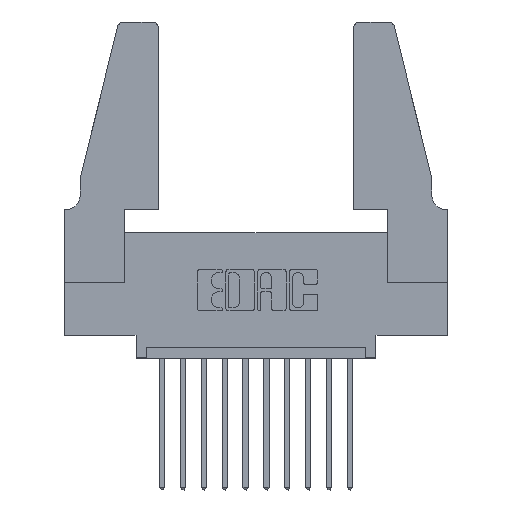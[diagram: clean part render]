
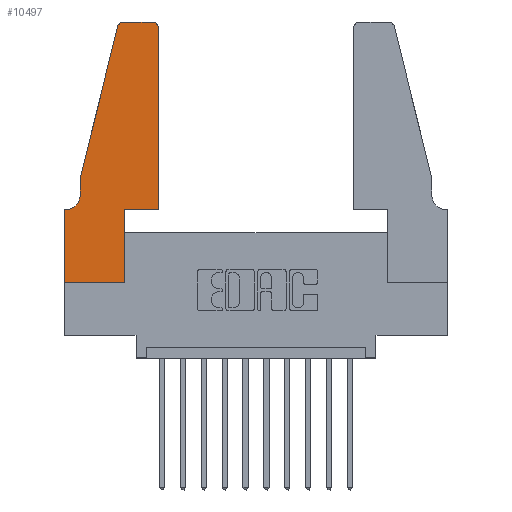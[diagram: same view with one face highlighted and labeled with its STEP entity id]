
A CAD part, top view. The second image highlights one B-rep face of the part: STEP entity #10497.
In plain terms, the highlighted planar face has unit normal (0, 0, 1).
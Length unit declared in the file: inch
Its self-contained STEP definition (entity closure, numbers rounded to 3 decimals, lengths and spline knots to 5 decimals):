
#153 = PLANE ( 'NONE',  #3836 ) ;
#181 = VERTEX_POINT ( 'NONE', #9110 ) ;
#348 = VERTEX_POINT ( 'NONE', #4529 ) ;
#361 = DIRECTION ( 'NONE',  ( 1., 0., 0. ) ) ;
#649 = DIRECTION ( 'NONE',  ( 0., -1., 0. ) ) ;
#734 = LINE ( 'NONE', #3218, #8589 ) ;
#907 = CARTESIAN_POINT ( 'NONE',  ( 0., 0., 0.37 ) ) ;
#1113 = EDGE_LOOP ( 'NONE', ( #7995, #12048, #8029, #8327, #5014, #5134, #14109, #6977, #10657, #8624, #7728, #1678 ) ) ;
#1229 = VECTOR ( 'NONE', #7771, 39.37008 ) ;
#1270 = CARTESIAN_POINT ( 'NONE',  ( 0., 0.35, 0.37 ) ) ;
#1297 = EDGE_CURVE ( 'NONE', #348, #7904, #1729, .T. ) ;
#1383 = VERTEX_POINT ( 'NONE', #4449 ) ;
#1439 = EDGE_CURVE ( 'NONE', #13309, #4636, #9750, .T. ) ;
#1475 = CARTESIAN_POINT ( 'NONE',  ( 0.4205, 1.25, 0.37 ) ) ;
#1489 = AXIS2_PLACEMENT_3D ( 'NONE', #8717, #2160, #9809 ) ;
#1678 = ORIENTED_EDGE ( 'NONE', *, *, #8527, .T. ) ;
#1729 = CIRCLE ( 'NONE', #1489, 0.07 ) ;
#1959 = CARTESIAN_POINT ( 'NONE',  ( 0.2605, 1.25, 0.37 ) ) ;
#2160 = DIRECTION ( 'NONE',  ( 0., 0., -1. ) ) ;
#2265 = AXIS2_PLACEMENT_3D ( 'NONE', #3436, #7798, #361 ) ;
#2539 = VECTOR ( 'NONE', #4648, 39.37008 ) ;
#3090 = VECTOR ( 'NONE', #8146, 39.37008 ) ;
#3218 = CARTESIAN_POINT ( 'NONE',  ( 0.2865, 0.35, 0.37 ) ) ;
#3329 = VERTEX_POINT ( 'NONE', #6638 ) ;
#3348 = CARTESIAN_POINT ( 'NONE',  ( 0., 0., 0.37 ) ) ;
#3436 = CARTESIAN_POINT ( 'NONE',  ( 0.4205, 1.22, 0.37 ) ) ;
#3503 = VECTOR ( 'NONE', #11050, 39.37008 ) ;
#3537 = CARTESIAN_POINT ( 'NONE',  ( 0.0755, 0.35, 0.37 ) ) ;
#3575 = LINE ( 'NONE', #3537, #2539 ) ;
#3617 = VERTEX_POINT ( 'NONE', #13131 ) ;
#3804 = VECTOR ( 'NONE', #9212, 39.37008 ) ;
#3836 = AXIS2_PLACEMENT_3D ( 'NONE', #1270, #4457, #8918 ) ;
#3867 = VERTEX_POINT ( 'NONE', #5359 ) ;
#4449 = CARTESIAN_POINT ( 'NONE',  ( 0.4505, 0.35, 0.37 ) ) ;
#4457 = DIRECTION ( 'NONE',  ( 0., 0., 1. ) ) ;
#4529 = CARTESIAN_POINT ( 'NONE',  ( 0.0755, 0.42, 0.37 ) ) ;
#4636 = VERTEX_POINT ( 'NONE', #9438 ) ;
#4648 = DIRECTION ( 'NONE',  ( -1., 0., 0. ) ) ;
#4811 = LINE ( 'NONE', #11480, #12326 ) ;
#5014 = ORIENTED_EDGE ( 'NONE', *, *, #1297, .T. ) ;
#5134 = ORIENTED_EDGE ( 'NONE', *, *, #10176, .T. ) ;
#5359 = CARTESIAN_POINT ( 'NONE',  ( 0.2865, 0.35, 0.37 ) ) ;
#5570 = CARTESIAN_POINT ( 'NONE',  ( 0.0755, 0.5, 0.37 ) ) ;
#5746 = EDGE_CURVE ( 'NONE', #9471, #3617, #8341, .T. ) ;
#5829 = EDGE_CURVE ( 'NONE', #9711, #9471, #8157, .T. ) ;
#5863 = EDGE_CURVE ( 'NONE', #11238, #13309, #10684, .T. ) ;
#6517 = DIRECTION ( 'NONE',  ( 0., -1., 0. ) ) ;
#6638 = CARTESIAN_POINT ( 'NONE',  ( 0.4505, 1.22, 0.37 ) ) ;
#6731 = LINE ( 'NONE', #9120, #3804 ) ;
#6977 = ORIENTED_EDGE ( 'NONE', *, *, #1439, .T. ) ;
#7017 = EDGE_CURVE ( 'NONE', #3617, #181, #8315, .T. ) ;
#7287 = DIRECTION ( 'NONE',  ( 1., 0., 0. ) ) ;
#7401 = CARTESIAN_POINT ( 'NONE',  ( 0., 0.35, 0.37 ) ) ;
#7728 = ORIENTED_EDGE ( 'NONE', *, *, #11634, .T. ) ;
#7771 = DIRECTION ( 'NONE',  ( 1., 0., 0. ) ) ;
#7798 = DIRECTION ( 'NONE',  ( 0., 0., 1. ) ) ;
#7818 = VECTOR ( 'NONE', #6517, 39.37008 ) ;
#7904 = VERTEX_POINT ( 'NONE', #11426 ) ;
#7995 = ORIENTED_EDGE ( 'NONE', *, *, #5829, .T. ) ;
#8029 = ORIENTED_EDGE ( 'NONE', *, *, #7017, .T. ) ;
#8146 = DIRECTION ( 'NONE',  ( 1., 0., 0. ) ) ;
#8157 = LINE ( 'NONE', #1959, #9852 ) ;
#8315 = LINE ( 'NONE', #5570, #3503 ) ;
#8327 = ORIENTED_EDGE ( 'NONE', *, *, #9731, .T. ) ;
#8341 = CIRCLE ( 'NONE', #9479, 0.03 ) ;
#8427 = CIRCLE ( 'NONE', #2265, 0.03 ) ;
#8449 = EDGE_CURVE ( 'NONE', #4636, #3867, #734, .T. ) ;
#8527 = EDGE_CURVE ( 'NONE', #3329, #9711, #8427, .T. ) ;
#8589 = VECTOR ( 'NONE', #8968, 39.37008 ) ;
#8612 = EDGE_CURVE ( 'NONE', #3867, #1383, #12013, .T. ) ;
#8624 = ORIENTED_EDGE ( 'NONE', *, *, #8612, .T. ) ;
#8717 = CARTESIAN_POINT ( 'NONE',  ( 0.0055, 0.42, 0.37 ) ) ;
#8918 = DIRECTION ( 'NONE',  ( 1., 0., 0. ) ) ;
#8968 = DIRECTION ( 'NONE',  ( 0., 1., 0. ) ) ;
#9110 = CARTESIAN_POINT ( 'NONE',  ( 0.0755, 0.5, 0.37 ) ) ;
#9120 = CARTESIAN_POINT ( 'NONE',  ( 0.4505, 0.35, 0.37 ) ) ;
#9212 = DIRECTION ( 'NONE',  ( 0., 1., 0. ) ) ;
#9438 = CARTESIAN_POINT ( 'NONE',  ( 0.2865, 0., 0.37 ) ) ;
#9471 = VERTEX_POINT ( 'NONE', #11413 ) ;
#9479 = AXIS2_PLACEMENT_3D ( 'NONE', #13777, #10417, #7287 ) ;
#9605 = DIRECTION ( 'NONE',  ( -1., 0., 0. ) ) ;
#9711 = VERTEX_POINT ( 'NONE', #1475 ) ;
#9731 = EDGE_CURVE ( 'NONE', #181, #348, #4811, .T. ) ;
#9750 = LINE ( 'NONE', #3348, #1229 ) ;
#9809 = DIRECTION ( 'NONE',  ( -1., 0., 0. ) ) ;
#9852 = VECTOR ( 'NONE', #9605, 39.37008 ) ;
#10176 = EDGE_CURVE ( 'NONE', #7904, #11238, #3575, .T. ) ;
#10417 = DIRECTION ( 'NONE',  ( 0., 0., 1. ) ) ;
#10497 = ADVANCED_FACE ( 'NONE', ( #11945 ), #153, .T. ) ;
#10657 = ORIENTED_EDGE ( 'NONE', *, *, #8449, .T. ) ;
#10684 = LINE ( 'NONE', #10824, #7818 ) ;
#10824 = CARTESIAN_POINT ( 'NONE',  ( 0., 0., 0.37 ) ) ;
#11050 = DIRECTION ( 'NONE',  ( -0.239, -0.971, 0. ) ) ;
#11238 = VERTEX_POINT ( 'NONE', #7401 ) ;
#11413 = CARTESIAN_POINT ( 'NONE',  ( 0.284, 1.25, 0.37 ) ) ;
#11426 = CARTESIAN_POINT ( 'NONE',  ( 0.0055, 0.35, 0.37 ) ) ;
#11437 = CARTESIAN_POINT ( 'NONE',  ( 0.4505, 0.35, 0.37 ) ) ;
#11480 = CARTESIAN_POINT ( 'NONE',  ( 0.0755, 0.5, 0.37 ) ) ;
#11634 = EDGE_CURVE ( 'NONE', #1383, #3329, #6731, .T. ) ;
#11945 = FACE_OUTER_BOUND ( 'NONE', #1113, .T. ) ;
#12013 = LINE ( 'NONE', #11437, #3090 ) ;
#12048 = ORIENTED_EDGE ( 'NONE', *, *, #5746, .T. ) ;
#12326 = VECTOR ( 'NONE', #649, 39.37008 ) ;
#13131 = CARTESIAN_POINT ( 'NONE',  ( 0.25487, 1.22718, 0.37 ) ) ;
#13309 = VERTEX_POINT ( 'NONE', #907 ) ;
#13777 = CARTESIAN_POINT ( 'NONE',  ( 0.284, 1.22, 0.37 ) ) ;
#14109 = ORIENTED_EDGE ( 'NONE', *, *, #5863, .T. ) ;
